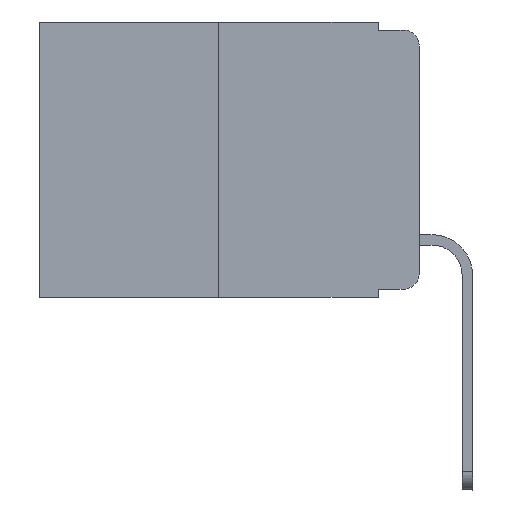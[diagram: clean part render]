
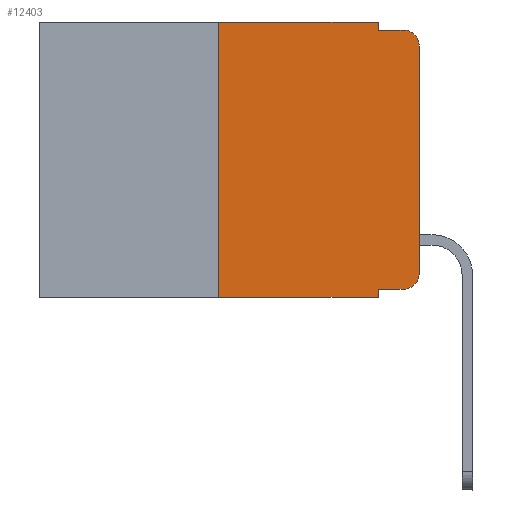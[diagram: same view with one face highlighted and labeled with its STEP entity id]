
A CAD part, left-side view. The second image highlights one B-rep face of the part: STEP entity #12403.
In plain terms, the highlighted planar face has unit normal (-1, 0, 0).
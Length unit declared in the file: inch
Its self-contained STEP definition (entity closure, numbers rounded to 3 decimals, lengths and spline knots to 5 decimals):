
#175 = CARTESIAN_POINT ( 'NONE',  ( 0., 0.473, 0. ) ) ;
#227 = AXIS2_PLACEMENT_3D ( 'NONE', #8077, #10397, #11784 ) ;
#273 = CARTESIAN_POINT ( 'NONE',  ( 0., 0.051, -0.333 ) ) ;
#285 = ORIENTED_EDGE ( 'NONE', *, *, #12903, .F. ) ;
#1344 = ORIENTED_EDGE ( 'NONE', *, *, #2321, .T. ) ;
#1532 = VERTEX_POINT ( 'NONE', #11459 ) ;
#1581 = CIRCLE ( 'NONE', #5757, 0.02 ) ;
#1618 = VECTOR ( 'NONE', #11969, 39.37008 ) ;
#1821 = VECTOR ( 'NONE', #3278, 39.37008 ) ;
#1859 = EDGE_CURVE ( 'NONE', #6308, #3783, #2127, .T. ) ;
#2067 = DIRECTION ( 'NONE',  ( 0., 0., -1. ) ) ;
#2127 = LINE ( 'NONE', #14894, #14752 ) ;
#2169 = ORIENTED_EDGE ( 'NONE', *, *, #1859, .F. ) ;
#2201 = VERTEX_POINT ( 'NONE', #4027 ) ;
#2321 = EDGE_CURVE ( 'NONE', #8211, #3783, #6972, .T. ) ;
#2838 = CARTESIAN_POINT ( 'NONE',  ( 0., 0.051, -0.333 ) ) ;
#3093 = LINE ( 'NONE', #4825, #12355 ) ;
#3153 = CARTESIAN_POINT ( 'NONE',  ( 0., 0.02, -0.313 ) ) ;
#3195 = VERTEX_POINT ( 'NONE', #8018 ) ;
#3197 = VECTOR ( 'NONE', #3948, 39.37008 ) ;
#3253 = CARTESIAN_POINT ( 'NONE',  ( 0., 0.051, 0. ) ) ;
#3278 = DIRECTION ( 'NONE',  ( 0., -1., 0. ) ) ;
#3375 = CARTESIAN_POINT ( 'NONE',  ( 0., 0.02, -0.01 ) ) ;
#3561 = ORIENTED_EDGE ( 'NONE', *, *, #13138, .F. ) ;
#3654 = ORIENTED_EDGE ( 'NONE', *, *, #9682, .T. ) ;
#3783 = VERTEX_POINT ( 'NONE', #7073 ) ;
#3796 = CARTESIAN_POINT ( 'NONE',  ( 0., 0.25, 0. ) ) ;
#3948 = DIRECTION ( 'NONE',  ( 0., -1., 0. ) ) ;
#4027 = CARTESIAN_POINT ( 'NONE',  ( 0., 0., -0.03 ) ) ;
#4229 = DIRECTION ( 'NONE',  ( 0., 0., -1. ) ) ;
#4532 = VERTEX_POINT ( 'NONE', #11063 ) ;
#4676 = ORIENTED_EDGE ( 'NONE', *, *, #6904, .F. ) ;
#4729 = VECTOR ( 'NONE', #4983, 39.37008 ) ;
#4825 = CARTESIAN_POINT ( 'NONE',  ( 0., 0., 0. ) ) ;
#4983 = DIRECTION ( 'NONE',  ( 0., -1., 0. ) ) ;
#5028 = ORIENTED_EDGE ( 'NONE', *, *, #5166, .F. ) ;
#5166 = EDGE_CURVE ( 'NONE', #1532, #6804, #7577, .T. ) ;
#5255 = LINE ( 'NONE', #3796, #16220 ) ;
#5369 = ORIENTED_EDGE ( 'NONE', *, *, #11428, .T. ) ;
#5461 = LINE ( 'NONE', #15506, #6823 ) ;
#5757 = AXIS2_PLACEMENT_3D ( 'NONE', #3153, #15909, #2067 ) ;
#5827 = CARTESIAN_POINT ( 'NONE',  ( 0., 0.473, -0.343 ) ) ;
#6223 = LINE ( 'NONE', #175, #4729 ) ;
#6308 = VERTEX_POINT ( 'NONE', #273 ) ;
#6478 = CARTESIAN_POINT ( 'NONE',  ( 0., 0.25, 0. ) ) ;
#6804 = VERTEX_POINT ( 'NONE', #3375 ) ;
#6823 = VECTOR ( 'NONE', #4229, 39.37008 ) ;
#6904 = EDGE_CURVE ( 'NONE', #8211, #7440, #5255, .T. ) ;
#6972 = LINE ( 'NONE', #5827, #1821 ) ;
#7073 = CARTESIAN_POINT ( 'NONE',  ( 0., 0.051, -0.343 ) ) ;
#7079 = FACE_OUTER_BOUND ( 'NONE', #9178, .T. ) ;
#7440 = VERTEX_POINT ( 'NONE', #6478 ) ;
#7577 = LINE ( 'NONE', #8972, #3197 ) ;
#8018 = CARTESIAN_POINT ( 'NONE',  ( 0., 0., -0.313 ) ) ;
#8077 = CARTESIAN_POINT ( 'NONE',  ( 0., 0.02, -0.03 ) ) ;
#8211 = VERTEX_POINT ( 'NONE', #16149 ) ;
#8972 = CARTESIAN_POINT ( 'NONE',  ( 0., 0.051, -0.01 ) ) ;
#9178 = EDGE_LOOP ( 'NONE', ( #5369, #3654, #5028, #3561, #285, #4676, #1344, #2169, #12360, #12927 ) ) ;
#9456 = AXIS2_PLACEMENT_3D ( 'NONE', #10631, #10963, #9645 ) ;
#9645 = DIRECTION ( 'NONE',  ( 0., 0., -1. ) ) ;
#9682 = EDGE_CURVE ( 'NONE', #2201, #6804, #16026, .T. ) ;
#10132 = DIRECTION ( 'NONE',  ( 0., 0., 1. ) ) ;
#10397 = DIRECTION ( 'NONE',  ( -1., 0., 0. ) ) ;
#10631 = CARTESIAN_POINT ( 'NONE',  ( 0., 0.473, 0. ) ) ;
#10963 = DIRECTION ( 'NONE',  ( 1., 0., 0. ) ) ;
#11063 = CARTESIAN_POINT ( 'NONE',  ( 0., 0.02, -0.333 ) ) ;
#11428 = EDGE_CURVE ( 'NONE', #3195, #2201, #3093, .T. ) ;
#11459 = CARTESIAN_POINT ( 'NONE',  ( 0., 0.051, -0.01 ) ) ;
#11784 = DIRECTION ( 'NONE',  ( 0., 0., -1. ) ) ;
#11923 = EDGE_CURVE ( 'NONE', #4532, #3195, #1581, .T. ) ;
#11969 = DIRECTION ( 'NONE',  ( 0., -1., 0. ) ) ;
#12229 = DIRECTION ( 'NONE',  ( 0., 0., 1. ) ) ;
#12355 = VECTOR ( 'NONE', #12229, 39.37008 ) ;
#12360 = ORIENTED_EDGE ( 'NONE', *, *, #14877, .T. ) ;
#12403 = ADVANCED_FACE ( 'NONE', ( #7079 ), #13504, .F. ) ;
#12903 = EDGE_CURVE ( 'NONE', #7440, #16088, #6223, .T. ) ;
#12927 = ORIENTED_EDGE ( 'NONE', *, *, #11923, .T. ) ;
#13138 = EDGE_CURVE ( 'NONE', #16088, #1532, #5461, .T. ) ;
#13504 = PLANE ( 'NONE',  #9456 ) ;
#14115 = LINE ( 'NONE', #2838, #1618 ) ;
#14752 = VECTOR ( 'NONE', #16127, 39.37008 ) ;
#14877 = EDGE_CURVE ( 'NONE', #6308, #4532, #14115, .T. ) ;
#14894 = CARTESIAN_POINT ( 'NONE',  ( 0., 0.051, 0. ) ) ;
#15506 = CARTESIAN_POINT ( 'NONE',  ( 0., 0.051, 0. ) ) ;
#15909 = DIRECTION ( 'NONE',  ( -1., 0., 0. ) ) ;
#16026 = CIRCLE ( 'NONE', #227, 0.02 ) ;
#16088 = VERTEX_POINT ( 'NONE', #3253 ) ;
#16127 = DIRECTION ( 'NONE',  ( 0., 0., -1. ) ) ;
#16149 = CARTESIAN_POINT ( 'NONE',  ( 0., 0.25, -0.343 ) ) ;
#16220 = VECTOR ( 'NONE', #10132, 39.37008 ) ;
